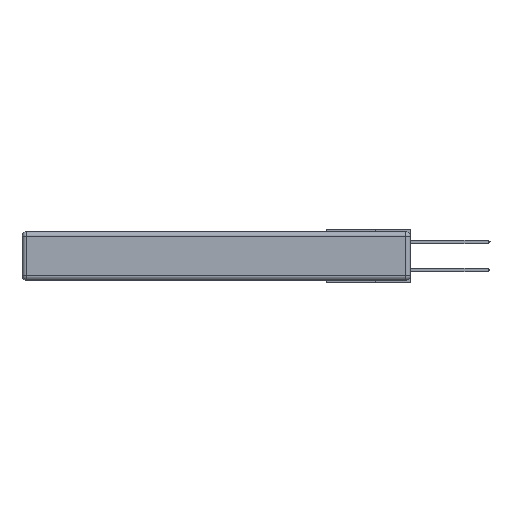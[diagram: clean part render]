
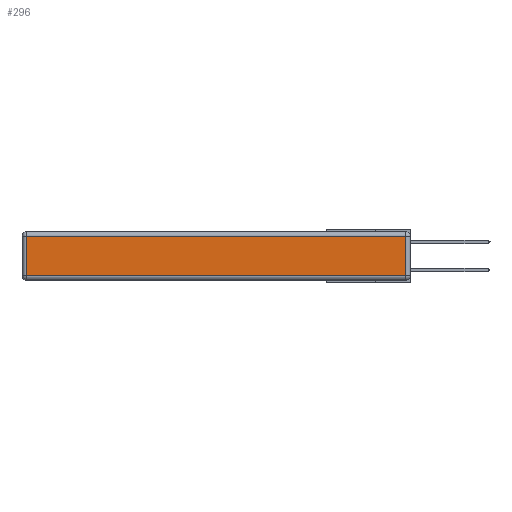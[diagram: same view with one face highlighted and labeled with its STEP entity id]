
A CAD part, left-side view. The second image highlights one B-rep face of the part: STEP entity #296.
In plain terms, the highlighted planar face has unit normal (-1, 0, 0).
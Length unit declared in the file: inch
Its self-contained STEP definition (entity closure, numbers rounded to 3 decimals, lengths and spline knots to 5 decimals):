
#188 = PLANE ( 'NONE',  #10050 ) ;
#296 = ADVANCED_FACE ( 'NONE', ( #5376 ), #188, .T. ) ;
#587 = VECTOR ( 'NONE', #3231, 39.37008 ) ;
#1083 = CARTESIAN_POINT ( 'NONE',  ( 0., 2.75, -0.03 ) ) ;
#1152 = VECTOR ( 'NONE', #11007, 39.37008 ) ;
#1506 = VERTEX_POINT ( 'NONE', #1904 ) ;
#1904 = CARTESIAN_POINT ( 'NONE',  ( 0., 2.72, -0.03 ) ) ;
#3045 = ORIENTED_EDGE ( 'NONE', *, *, #3898, .T. ) ;
#3110 = LINE ( 'NONE', #7203, #587 ) ;
#3209 = DIRECTION ( 'NONE',  ( 0., 1., 0. ) ) ;
#3231 = DIRECTION ( 'NONE',  ( 0., 0., -1. ) ) ;
#3347 = DIRECTION ( 'NONE',  ( 0., 0., 1. ) ) ;
#3383 = EDGE_CURVE ( 'NONE', #13932, #1506, #4454, .T. ) ;
#3392 = DIRECTION ( 'NONE',  ( -1., 0., 0. ) ) ;
#3898 = EDGE_CURVE ( 'NONE', #1506, #12983, #3110, .T. ) ;
#3931 = VECTOR ( 'NONE', #8896, 39.37008 ) ;
#4454 = LINE ( 'NONE', #1083, #10444 ) ;
#4943 = LINE ( 'NONE', #7847, #3931 ) ;
#5376 = FACE_OUTER_BOUND ( 'NONE', #13311, .T. ) ;
#5537 = LINE ( 'NONE', #11105, #1152 ) ;
#5544 = CARTESIAN_POINT ( 'NONE',  ( 0., 2.72, -0.313 ) ) ;
#5582 = CARTESIAN_POINT ( 'NONE',  ( 0., 0.03, -0.03 ) ) ;
#7203 = CARTESIAN_POINT ( 'NONE',  ( 0., 2.72, -0.343 ) ) ;
#7453 = EDGE_CURVE ( 'NONE', #10890, #13932, #4943, .T. ) ;
#7847 = CARTESIAN_POINT ( 'NONE',  ( 0., 0.03, -0.343 ) ) ;
#8896 = DIRECTION ( 'NONE',  ( 0., 0., 1. ) ) ;
#9263 = CARTESIAN_POINT ( 'NONE',  ( 0., 0.03, -0.313 ) ) ;
#9898 = CARTESIAN_POINT ( 'NONE',  ( 0., 0., -0.343 ) ) ;
#10050 = AXIS2_PLACEMENT_3D ( 'NONE', #9898, #3392, #3347 ) ;
#10390 = EDGE_CURVE ( 'NONE', #12983, #10890, #5537, .T. ) ;
#10444 = VECTOR ( 'NONE', #3209, 39.37008 ) ;
#10890 = VERTEX_POINT ( 'NONE', #9263 ) ;
#11007 = DIRECTION ( 'NONE',  ( 0., -1., 0. ) ) ;
#11105 = CARTESIAN_POINT ( 'NONE',  ( 0., 0., -0.313 ) ) ;
#11646 = ORIENTED_EDGE ( 'NONE', *, *, #7453, .T. ) ;
#12400 = ORIENTED_EDGE ( 'NONE', *, *, #10390, .T. ) ;
#12960 = ORIENTED_EDGE ( 'NONE', *, *, #3383, .T. ) ;
#12983 = VERTEX_POINT ( 'NONE', #5544 ) ;
#13311 = EDGE_LOOP ( 'NONE', ( #12400, #11646, #12960, #3045 ) ) ;
#13932 = VERTEX_POINT ( 'NONE', #5582 ) ;
